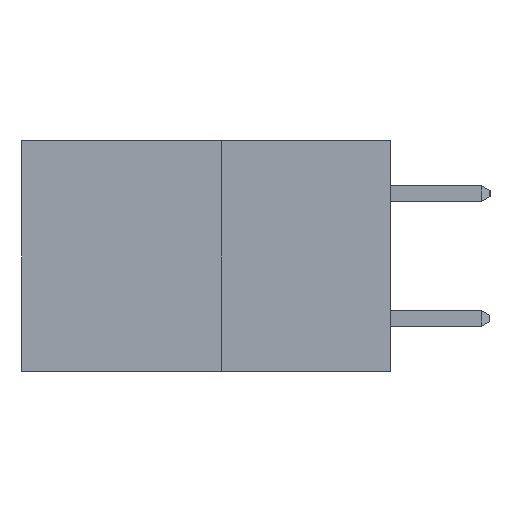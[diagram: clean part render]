
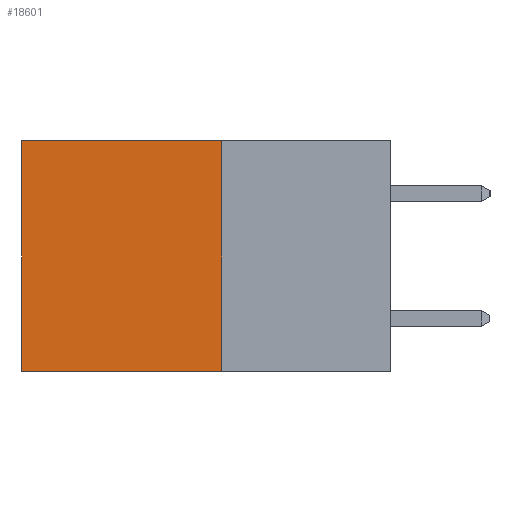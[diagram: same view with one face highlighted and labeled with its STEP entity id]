
A CAD part, left-side view. The second image highlights one B-rep face of the part: STEP entity #18601.
In plain terms, the highlighted planar face has unit normal (-1, 0, 0).
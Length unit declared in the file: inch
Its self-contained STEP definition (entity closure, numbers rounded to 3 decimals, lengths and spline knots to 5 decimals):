
#26 = VERTEX_POINT ( 'NONE', #21609 ) ;
#631 = LINE ( 'NONE', #13400, #9377 ) ;
#862 = CARTESIAN_POINT ( 'NONE',  ( 0.277, 0.27, -0.37 ) ) ;
#2405 = EDGE_CURVE ( 'NONE', #3862, #26, #20502, .T. ) ;
#2704 = VECTOR ( 'NONE', #17507, 39.37008 ) ;
#2818 = ORIENTED_EDGE ( 'NONE', *, *, #4382, .T. ) ;
#2942 = CARTESIAN_POINT ( 'NONE',  ( 0.277, 0.59, -0.37 ) ) ;
#3862 = VERTEX_POINT ( 'NONE', #6368 ) ;
#4382 = EDGE_CURVE ( 'NONE', #3862, #19339, #13159, .T. ) ;
#4484 = ORIENTED_EDGE ( 'NONE', *, *, #8120, .F. ) ;
#4626 = FACE_OUTER_BOUND ( 'NONE', #6300, .T. ) ;
#5686 = LINE ( 'NONE', #2942, #18856 ) ;
#6300 = EDGE_LOOP ( 'NONE', ( #16343, #4484, #10151, #2818 ) ) ;
#6368 = CARTESIAN_POINT ( 'NONE',  ( 0.277, 0.27, 0. ) ) ;
#6455 = DIRECTION ( 'NONE',  ( 0., 0., -1. ) ) ;
#7142 = DIRECTION ( 'NONE',  ( 0., 0., -1. ) ) ;
#7987 = AXIS2_PLACEMENT_3D ( 'NONE', #15717, #17443, #7142 ) ;
#8120 = EDGE_CURVE ( 'NONE', #26, #12682, #631, .T. ) ;
#8591 = VECTOR ( 'NONE', #13202, 39.37008 ) ;
#9377 = VECTOR ( 'NONE', #15140, 39.37008 ) ;
#10151 = ORIENTED_EDGE ( 'NONE', *, *, #2405, .F. ) ;
#11929 = CARTESIAN_POINT ( 'NONE',  ( 0.277, 0.59, -0.37 ) ) ;
#12682 = VERTEX_POINT ( 'NONE', #11929 ) ;
#13159 = LINE ( 'NONE', #13196, #8591 ) ;
#13196 = CARTESIAN_POINT ( 'NONE',  ( 0.277, 0.27, 0. ) ) ;
#13202 = DIRECTION ( 'NONE',  ( 0., 1., 0. ) ) ;
#13400 = CARTESIAN_POINT ( 'NONE',  ( 0.277, 0.27, -0.37 ) ) ;
#13964 = PLANE ( 'NONE',  #7987 ) ;
#15140 = DIRECTION ( 'NONE',  ( 0., 1., 0. ) ) ;
#15717 = CARTESIAN_POINT ( 'NONE',  ( 0.277, 0.27, -0.37 ) ) ;
#16343 = ORIENTED_EDGE ( 'NONE', *, *, #16908, .T. ) ;
#16908 = EDGE_CURVE ( 'NONE', #19339, #12682, #5686, .T. ) ;
#17443 = DIRECTION ( 'NONE',  ( 1., 0., 0. ) ) ;
#17507 = DIRECTION ( 'NONE',  ( 0., 0., -1. ) ) ;
#17944 = CARTESIAN_POINT ( 'NONE',  ( 0.277, 0.59, 0. ) ) ;
#18601 = ADVANCED_FACE ( 'NONE', ( #4626 ), #13964, .F. ) ;
#18856 = VECTOR ( 'NONE', #6455, 39.37008 ) ;
#19339 = VERTEX_POINT ( 'NONE', #17944 ) ;
#20502 = LINE ( 'NONE', #862, #2704 ) ;
#21609 = CARTESIAN_POINT ( 'NONE',  ( 0.277, 0.27, -0.37 ) ) ;
